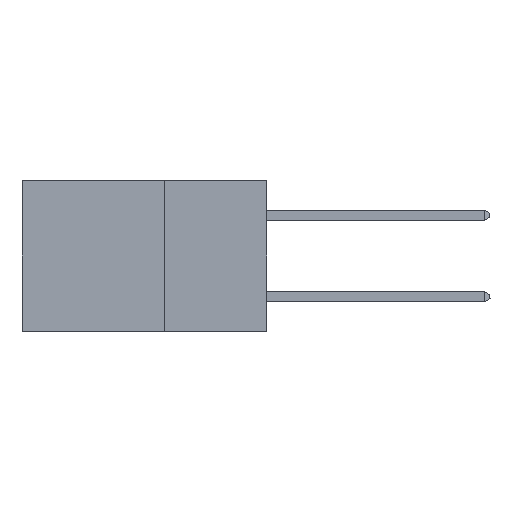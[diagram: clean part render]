
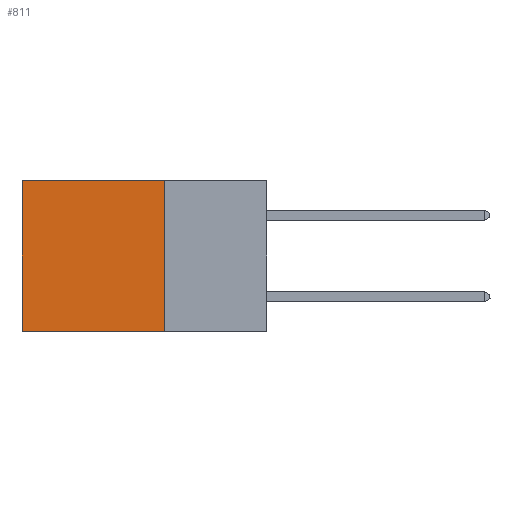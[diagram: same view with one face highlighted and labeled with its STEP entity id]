
A CAD part, left-side view. The second image highlights one B-rep face of the part: STEP entity #811.
In plain terms, the highlighted planar face has unit normal (-1, 0, 0).
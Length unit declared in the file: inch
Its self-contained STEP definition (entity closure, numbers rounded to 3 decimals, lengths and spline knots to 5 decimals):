
#716 = AXIS2_PLACEMENT_3D ( 'NONE', #9888, #9725, #6294 ) ;
#811 = ADVANCED_FACE ( 'NONE', ( #21851 ), #20025, .F. ) ;
#3264 = VECTOR ( 'NONE', #21066, 39.37008 ) ;
#3940 = EDGE_CURVE ( 'NONE', #13754, #3995, #5539, .T. ) ;
#3995 = VERTEX_POINT ( 'NONE', #21807 ) ;
#4493 = ORIENTED_EDGE ( 'NONE', *, *, #7912, .F. ) ;
#4771 = ORIENTED_EDGE ( 'NONE', *, *, #14318, .T. ) ;
#5539 = LINE ( 'NONE', #21523, #15662 ) ;
#5553 = VERTEX_POINT ( 'NONE', #16890 ) ;
#6294 = DIRECTION ( 'NONE',  ( 0., 0., -1. ) ) ;
#6845 = EDGE_CURVE ( 'NONE', #5553, #7136, #21101, .T. ) ;
#7136 = VERTEX_POINT ( 'NONE', #21121 ) ;
#7912 = EDGE_CURVE ( 'NONE', #3995, #7136, #8591, .T. ) ;
#8523 = CARTESIAN_POINT ( 'NONE',  ( 0.2875, 0.6, 0. ) ) ;
#8591 = LINE ( 'NONE', #16842, #20541 ) ;
#9725 = DIRECTION ( 'NONE',  ( 1., 0., 0. ) ) ;
#9888 = CARTESIAN_POINT ( 'NONE',  ( 0.2875, 0.25, 0. ) ) ;
#11538 = LINE ( 'NONE', #17682, #3264 ) ;
#13754 = VERTEX_POINT ( 'NONE', #18838 ) ;
#14109 = DIRECTION ( 'NONE',  ( 0., 0., -1. ) ) ;
#14318 = EDGE_CURVE ( 'NONE', #13754, #5553, #11538, .T. ) ;
#14887 = DIRECTION ( 'NONE',  ( 0., 0., -1. ) ) ;
#15061 = DIRECTION ( 'NONE',  ( 0., 1., 0. ) ) ;
#15662 = VECTOR ( 'NONE', #14887, 39.37008 ) ;
#16363 = VECTOR ( 'NONE', #14109, 39.37008 ) ;
#16842 = CARTESIAN_POINT ( 'NONE',  ( 0.2875, 0.25, -0.37 ) ) ;
#16890 = CARTESIAN_POINT ( 'NONE',  ( 0.2875, 0.6, 0. ) ) ;
#17682 = CARTESIAN_POINT ( 'NONE',  ( 0.2875, 0.25, 0. ) ) ;
#18838 = CARTESIAN_POINT ( 'NONE',  ( 0.2875, 0.25, 0. ) ) ;
#19265 = ORIENTED_EDGE ( 'NONE', *, *, #3940, .F. ) ;
#20025 = PLANE ( 'NONE',  #716 ) ;
#20541 = VECTOR ( 'NONE', #15061, 39.37008 ) ;
#21066 = DIRECTION ( 'NONE',  ( 0., 1., 0. ) ) ;
#21101 = LINE ( 'NONE', #8523, #16363 ) ;
#21121 = CARTESIAN_POINT ( 'NONE',  ( 0.2875, 0.6, -0.37 ) ) ;
#21523 = CARTESIAN_POINT ( 'NONE',  ( 0.2875, 0.25, 0. ) ) ;
#21660 = ORIENTED_EDGE ( 'NONE', *, *, #6845, .T. ) ;
#21736 = EDGE_LOOP ( 'NONE', ( #21660, #4493, #19265, #4771 ) ) ;
#21807 = CARTESIAN_POINT ( 'NONE',  ( 0.2875, 0.25, -0.37 ) ) ;
#21851 = FACE_OUTER_BOUND ( 'NONE', #21736, .T. ) ;
